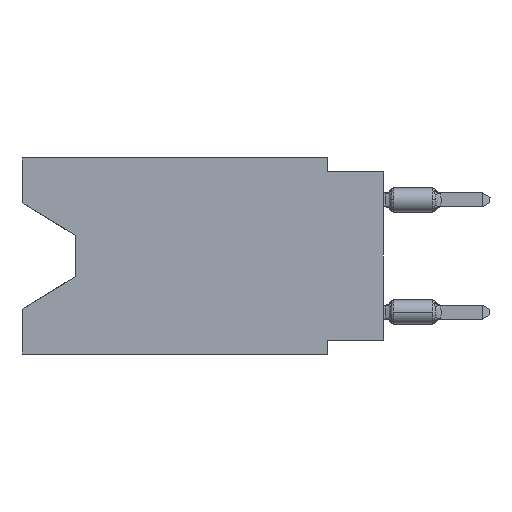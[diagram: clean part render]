
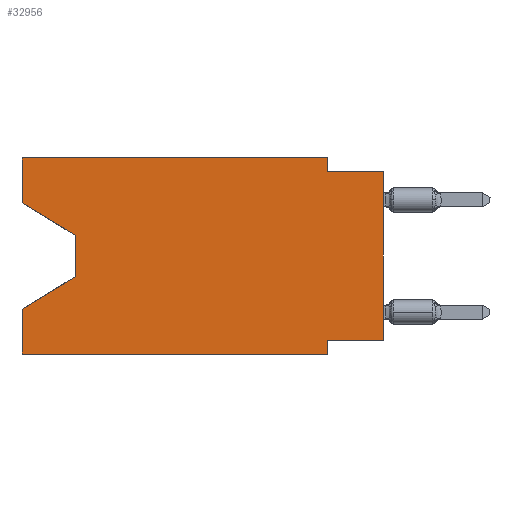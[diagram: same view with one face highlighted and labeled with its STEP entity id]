
A CAD part, left-side view. The second image highlights one B-rep face of the part: STEP entity #32956.
In plain terms, the highlighted planar face has unit normal (-1, 0, 0).
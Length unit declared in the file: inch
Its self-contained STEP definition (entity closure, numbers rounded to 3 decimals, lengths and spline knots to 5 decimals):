
#619 = CARTESIAN_POINT ( 'NONE',  ( 0., 0.55, -0.138 ) ) ;
#969 = CARTESIAN_POINT ( 'NONE',  ( 0., 0., -0.325 ) ) ;
#1034 = VERTEX_POINT ( 'NONE', #619 ) ;
#1672 = LINE ( 'NONE', #7569, #27730 ) ;
#1876 = VERTEX_POINT ( 'NONE', #6069 ) ;
#2102 = DIRECTION ( 'NONE',  ( 0., -1., 0. ) ) ;
#2182 = CARTESIAN_POINT ( 'NONE',  ( 0., 0.645, -0.35 ) ) ;
#2232 = CARTESIAN_POINT ( 'NONE',  ( 0., 0.1, 0. ) ) ;
#3658 = VECTOR ( 'NONE', #8438, 39.37008 ) ;
#4081 = DIRECTION ( 'NONE',  ( 0., 0., -1. ) ) ;
#4236 = ORIENTED_EDGE ( 'NONE', *, *, #37221, .F. ) ;
#4258 = CARTESIAN_POINT ( 'NONE',  ( 0., 0.645, 0. ) ) ;
#4310 = CARTESIAN_POINT ( 'NONE',  ( 0., 0.645, -0.08025 ) ) ;
#4388 = CARTESIAN_POINT ( 'NONE',  ( 0., 0.1, -0.35 ) ) ;
#4583 = ORIENTED_EDGE ( 'NONE', *, *, #8046, .F. ) ;
#4677 = DIRECTION ( 'NONE',  ( 0., 0., -1. ) ) ;
#5473 = VECTOR ( 'NONE', #26052, 39.37008 ) ;
#5937 = ORIENTED_EDGE ( 'NONE', *, *, #25456, .T. ) ;
#6069 = CARTESIAN_POINT ( 'NONE',  ( 0., 0.645, -0.08025 ) ) ;
#6356 = ORIENTED_EDGE ( 'NONE', *, *, #18354, .F. ) ;
#7380 = VERTEX_POINT ( 'NONE', #26266 ) ;
#7537 = CARTESIAN_POINT ( 'NONE',  ( 0., 0.1, -0.35 ) ) ;
#7569 = CARTESIAN_POINT ( 'NONE',  ( 0., 0.55, -0.138 ) ) ;
#7655 = CARTESIAN_POINT ( 'NONE',  ( 0., 0.1, 0. ) ) ;
#8046 = EDGE_CURVE ( 'NONE', #20127, #22187, #21706, .T. ) ;
#8213 = DIRECTION ( 'NONE',  ( 0., 0.855, -0.519 ) ) ;
#8438 = DIRECTION ( 'NONE',  ( 0., -0.855, -0.519 ) ) ;
#8796 = EDGE_CURVE ( 'NONE', #1034, #36638, #1672, .T. ) ;
#8956 = ORIENTED_EDGE ( 'NONE', *, *, #16582, .F. ) ;
#9053 = DIRECTION ( 'NONE',  ( 0., 0., 1. ) ) ;
#9527 = CARTESIAN_POINT ( 'NONE',  ( 0., 0., -0.025 ) ) ;
#10151 = CARTESIAN_POINT ( 'NONE',  ( 0., 0.1, -0.025 ) ) ;
#10224 = VERTEX_POINT ( 'NONE', #2182 ) ;
#10454 = EDGE_CURVE ( 'NONE', #1876, #20127, #33542, .T. ) ;
#10509 = VECTOR ( 'NONE', #2102, 39.37008 ) ;
#11422 = VERTEX_POINT ( 'NONE', #33397 ) ;
#12343 = VECTOR ( 'NONE', #36412, 39.37008 ) ;
#12585 = DIRECTION ( 'NONE',  ( 0., 1., 0. ) ) ;
#12867 = EDGE_CURVE ( 'NONE', #36638, #20517, #31253, .T. ) ;
#12910 = VECTOR ( 'NONE', #16834, 39.37008 ) ;
#13223 = FACE_OUTER_BOUND ( 'NONE', #17869, .T. ) ;
#14249 = ORIENTED_EDGE ( 'NONE', *, *, #12867, .T. ) ;
#14660 = LINE ( 'NONE', #29139, #25670 ) ;
#15119 = ORIENTED_EDGE ( 'NONE', *, *, #16145, .F. ) ;
#15431 = LINE ( 'NONE', #969, #16258 ) ;
#15826 = AXIS2_PLACEMENT_3D ( 'NONE', #4258, #30172, #4081 ) ;
#16145 = EDGE_CURVE ( 'NONE', #11422, #7380, #15431, .T. ) ;
#16258 = VECTOR ( 'NONE', #12585, 39.37008 ) ;
#16582 = EDGE_CURVE ( 'NONE', #7380, #21377, #21808, .T. ) ;
#16834 = DIRECTION ( 'NONE',  ( 0., -1., 0. ) ) ;
#17039 = CARTESIAN_POINT ( 'NONE',  ( 0., 0.55, -0.212 ) ) ;
#17869 = EDGE_LOOP ( 'NONE', ( #5937, #27426, #14249, #27335, #35306, #8956, #15119, #19602, #6356, #4236, #4583, #26010 ) ) ;
#18354 = EDGE_CURVE ( 'NONE', #26874, #22033, #20066, .T. ) ;
#18822 = CARTESIAN_POINT ( 'NONE',  ( 0., 0.645, 0. ) ) ;
#19051 = CARTESIAN_POINT ( 'NONE',  ( 0., 0.645, 0. ) ) ;
#19602 = ORIENTED_EDGE ( 'NONE', *, *, #34566, .T. ) ;
#19803 = CARTESIAN_POINT ( 'NONE',  ( 0., 0.55, -0.212 ) ) ;
#19846 = LINE ( 'NONE', #4310, #3658 ) ;
#20066 = LINE ( 'NONE', #34561, #12910 ) ;
#20127 = VERTEX_POINT ( 'NONE', #22582 ) ;
#20517 = VERTEX_POINT ( 'NONE', #21426 ) ;
#20841 = LINE ( 'NONE', #29608, #28131 ) ;
#21377 = VERTEX_POINT ( 'NONE', #4388 ) ;
#21426 = CARTESIAN_POINT ( 'NONE',  ( 0., 0.645, -0.26975 ) ) ;
#21706 = LINE ( 'NONE', #18822, #10509 ) ;
#21808 = LINE ( 'NONE', #7537, #31235 ) ;
#22033 = VERTEX_POINT ( 'NONE', #9527 ) ;
#22187 = VERTEX_POINT ( 'NONE', #2232 ) ;
#22582 = CARTESIAN_POINT ( 'NONE',  ( 0., 0.645, 0. ) ) ;
#25171 = VECTOR ( 'NONE', #28015, 39.37008 ) ;
#25456 = EDGE_CURVE ( 'NONE', #1876, #1034, #19846, .T. ) ;
#25670 = VECTOR ( 'NONE', #35064, 39.37008 ) ;
#26010 = ORIENTED_EDGE ( 'NONE', *, *, #10454, .F. ) ;
#26052 = DIRECTION ( 'NONE',  ( 0., -1., 0. ) ) ;
#26266 = CARTESIAN_POINT ( 'NONE',  ( 0., 0.1, -0.325 ) ) ;
#26874 = VERTEX_POINT ( 'NONE', #10151 ) ;
#27335 = ORIENTED_EDGE ( 'NONE', *, *, #36692, .F. ) ;
#27426 = ORIENTED_EDGE ( 'NONE', *, *, #8796, .T. ) ;
#27730 = VECTOR ( 'NONE', #33837, 39.37008 ) ;
#28015 = DIRECTION ( 'NONE',  ( 0., 0., 1. ) ) ;
#28131 = VECTOR ( 'NONE', #9053, 39.37008 ) ;
#29083 = CARTESIAN_POINT ( 'NONE',  ( 0., 0.645, -0.35 ) ) ;
#29139 = CARTESIAN_POINT ( 'NONE',  ( 0., 0., 0. ) ) ;
#29570 = VECTOR ( 'NONE', #8213, 39.37008 ) ;
#29608 = CARTESIAN_POINT ( 'NONE',  ( 0., 0.645, 0. ) ) ;
#30172 = DIRECTION ( 'NONE',  ( 1., 0., 0. ) ) ;
#31235 = VECTOR ( 'NONE', #4677, 39.37008 ) ;
#31253 = LINE ( 'NONE', #19803, #29570 ) ;
#31957 = LINE ( 'NONE', #29083, #5473 ) ;
#32213 = EDGE_CURVE ( 'NONE', #10224, #21377, #31957, .T. ) ;
#32956 = ADVANCED_FACE ( 'NONE', ( #13223 ), #33019, .F. ) ;
#33019 = PLANE ( 'NONE',  #15826 ) ;
#33169 = LINE ( 'NONE', #7655, #12343 ) ;
#33397 = CARTESIAN_POINT ( 'NONE',  ( 0., 0., -0.325 ) ) ;
#33542 = LINE ( 'NONE', #19051, #25171 ) ;
#33837 = DIRECTION ( 'NONE',  ( 0., 0., -1. ) ) ;
#34561 = CARTESIAN_POINT ( 'NONE',  ( 0., 0., -0.025 ) ) ;
#34566 = EDGE_CURVE ( 'NONE', #11422, #22033, #14660, .T. ) ;
#35064 = DIRECTION ( 'NONE',  ( 0., 0., 1. ) ) ;
#35306 = ORIENTED_EDGE ( 'NONE', *, *, #32213, .T. ) ;
#36412 = DIRECTION ( 'NONE',  ( 0., 0., -1. ) ) ;
#36638 = VERTEX_POINT ( 'NONE', #17039 ) ;
#36692 = EDGE_CURVE ( 'NONE', #10224, #20517, #20841, .T. ) ;
#37221 = EDGE_CURVE ( 'NONE', #22187, #26874, #33169, .T. ) ;
